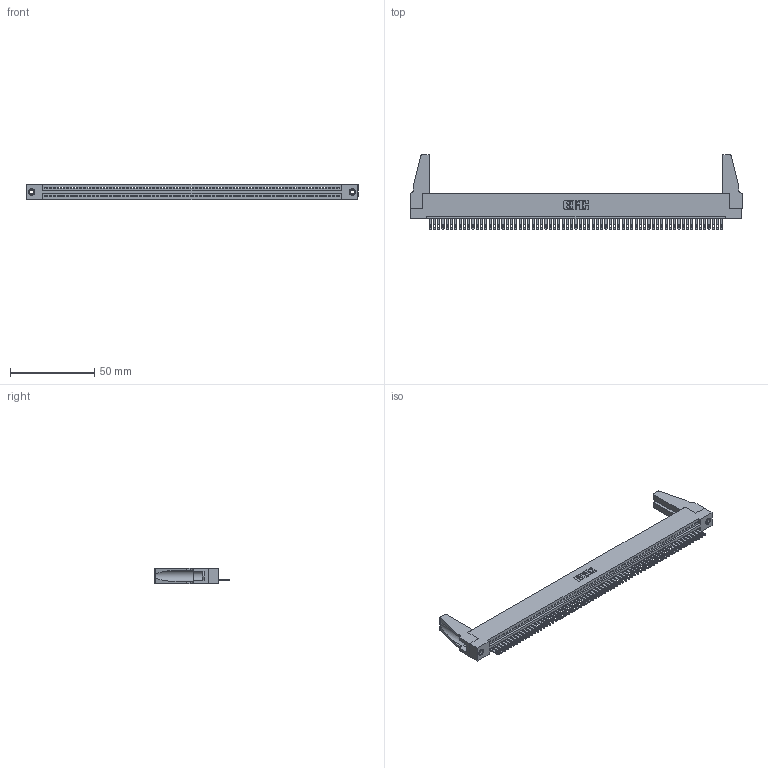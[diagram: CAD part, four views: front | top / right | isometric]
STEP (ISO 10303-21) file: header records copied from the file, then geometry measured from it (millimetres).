
FILE_DESCRIPTION (( 'STEP AP203' ), '1' );
FILE_NAME ('345-069-500-188.STEP', '2019-10-12T08:45:11', ( '' ), ( '' ), 'SwSTEP 2.0', 'SolidWorks 2016', '' );
FILE_SCHEMA (( 'CONFIG_CONTROL_DESIGN' ));
Length unit declared in the file: inch
Products named in the file (5): 345-292-001_345-293-100; 345-220-078_345-220-088; 345-250-001_345-250-001-102; 345 Part_Flush Mounting Lugs - 0.156 Dia-TH; 345-069-500-188
Assembly tree (74 placements, depth 2):
  345-069-500-188
    345 Part_Flush Mounting Lugs - 0.156 Dia-TH
    345-292-001_345-293-100  x69
    345-250-001_345-250-001-102  x2
    345-220-078_345-220-088  x2
Bounding box: 196.49 x 44.37 x 9.4 mm (x, y, z)
Volume: 22179.6 mm3; surface area: 28803.6 mm2
Topology: 74 solids, 74 shells, 3976 faces, 12247 edges, 8154 vertices
Faces by surface type: plane 2498, cylinder 1462, cone 12, torus 4
Entity records: 50374 total; most frequent: CARTESIAN_POINT 8713, ORIENTED_EDGE 8676, DIRECTION 7580, EDGE_CURVE 4338, VECTOR 3884, LINE 3884, VERTEX_POINT 2886, AXIS2_PLACEMENT_3D 1848
